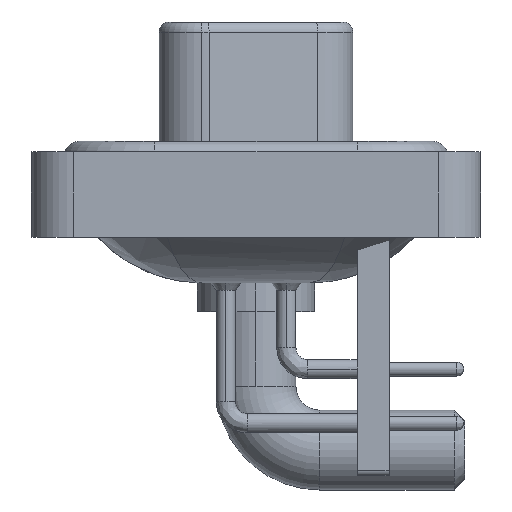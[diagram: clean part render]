
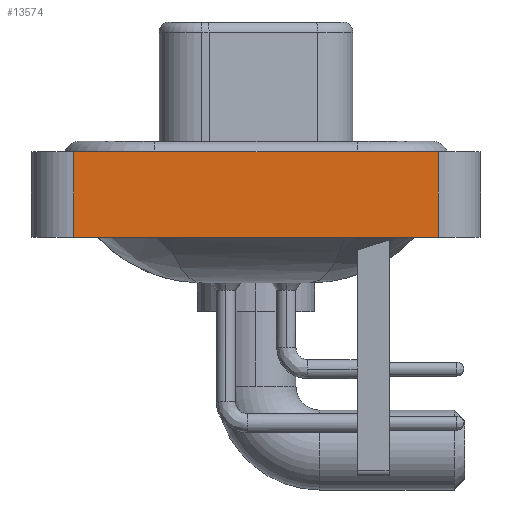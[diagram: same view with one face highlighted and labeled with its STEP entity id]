
A CAD part, left-side view. The second image highlights one B-rep face of the part: STEP entity #13574.
In plain terms, the highlighted planar face has unit normal (-1, 0, 0).
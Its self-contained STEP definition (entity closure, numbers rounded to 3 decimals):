
#314 = DIRECTION ( 'NONE',  ( 0., -1., 0. ) ) ;
#1145 = LINE ( 'NONE', #6650, #20029 ) ;
#1479 = AXIS2_PLACEMENT_3D ( 'NONE', #16836, #9444, #18650 ) ;
#1483 = CARTESIAN_POINT ( 'NONE',  ( -7.25, 8.55, 0.4 ) ) ;
#1562 = CARTESIAN_POINT ( 'NONE',  ( -7.25, 8.55, -3.6 ) ) ;
#1583 = VECTOR ( 'NONE', #21888, 1000. ) ;
#2705 = VERTEX_POINT ( 'NONE', #1483 ) ;
#3370 = LINE ( 'NONE', #1562, #1583 ) ;
#3784 = CARTESIAN_POINT ( 'NONE',  ( -7.25, -8.55, 0.4 ) ) ;
#4100 = CARTESIAN_POINT ( 'NONE',  ( -7.25, -8.55, -3.6 ) ) ;
#4759 = ORIENTED_EDGE ( 'NONE', *, *, #18187, .T. ) ;
#6650 = CARTESIAN_POINT ( 'NONE',  ( -7.25, -8.55, 0.4 ) ) ;
#9444 = DIRECTION ( 'NONE',  ( -1., 0., 0. ) ) ;
#9447 = VECTOR ( 'NONE', #314, 1000. ) ;
#10139 = LINE ( 'NONE', #16954, #12531 ) ;
#11623 = EDGE_CURVE ( 'NONE', #2705, #16777, #1145, .T. ) ;
#12320 = VERTEX_POINT ( 'NONE', #18660 ) ;
#12531 = VECTOR ( 'NONE', #20904, 1000. ) ;
#13339 = LINE ( 'NONE', #20630, #9447 ) ;
#13574 = ADVANCED_FACE ( 'NONE', ( #20442 ), #18522, .T. ) ;
#13823 = EDGE_CURVE ( 'NONE', #23160, #16777, #10139, .T. ) ;
#15404 = ORIENTED_EDGE ( 'NONE', *, *, #11623, .F. ) ;
#15893 = EDGE_CURVE ( 'NONE', #12320, #2705, #3370, .T. ) ;
#16054 = EDGE_LOOP ( 'NONE', ( #16228, #15404, #22050, #4759 ) ) ;
#16228 = ORIENTED_EDGE ( 'NONE', *, *, #13823, .T. ) ;
#16777 = VERTEX_POINT ( 'NONE', #3784 ) ;
#16836 = CARTESIAN_POINT ( 'NONE',  ( -7.25, -8.55, -3.6 ) ) ;
#16954 = CARTESIAN_POINT ( 'NONE',  ( -7.25, -8.55, -3.6 ) ) ;
#18187 = EDGE_CURVE ( 'NONE', #12320, #23160, #13339, .T. ) ;
#18522 = PLANE ( 'NONE',  #1479 ) ;
#18650 = DIRECTION ( 'NONE',  ( 0., 0., 1. ) ) ;
#18660 = CARTESIAN_POINT ( 'NONE',  ( -7.25, 8.55, -3.6 ) ) ;
#20029 = VECTOR ( 'NONE', #21831, 1000. ) ;
#20442 = FACE_OUTER_BOUND ( 'NONE', #16054, .T. ) ;
#20630 = CARTESIAN_POINT ( 'NONE',  ( -7.25, -8.55, -3.6 ) ) ;
#20904 = DIRECTION ( 'NONE',  ( 0., 0., 1. ) ) ;
#21831 = DIRECTION ( 'NONE',  ( 0., -1., 0. ) ) ;
#21888 = DIRECTION ( 'NONE',  ( 0., 0., 1. ) ) ;
#22050 = ORIENTED_EDGE ( 'NONE', *, *, #15893, .F. ) ;
#23160 = VERTEX_POINT ( 'NONE', #4100 ) ;
